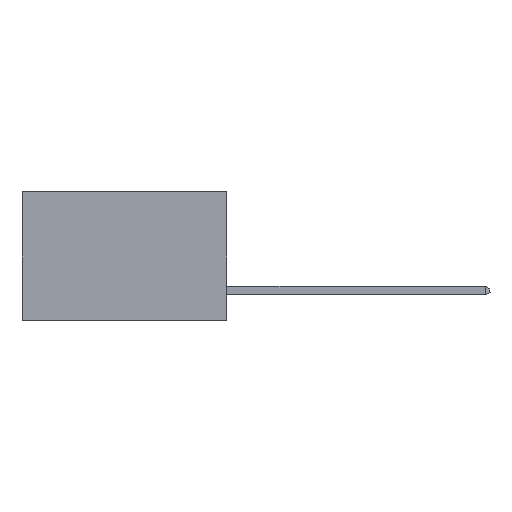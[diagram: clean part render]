
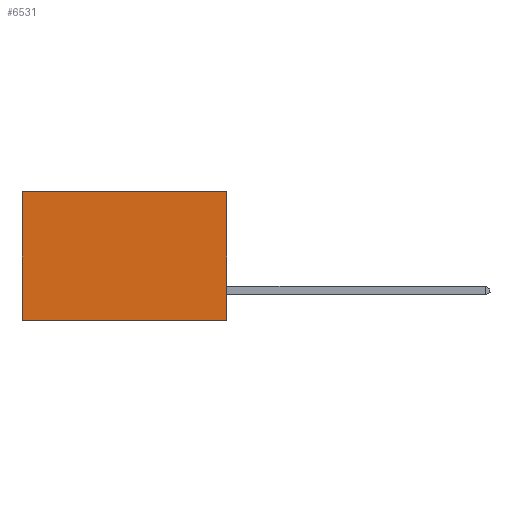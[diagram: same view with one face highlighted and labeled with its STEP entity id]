
A CAD part, left-side view. The second image highlights one B-rep face of the part: STEP entity #6531.
In plain terms, the highlighted planar face has unit normal (-1, 0, 0).
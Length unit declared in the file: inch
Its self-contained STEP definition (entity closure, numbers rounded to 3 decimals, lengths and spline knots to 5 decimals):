
#491 = EDGE_CURVE ( 'NONE', #18198, #8046, #5920, .T. ) ;
#566 = ORIENTED_EDGE ( 'NONE', *, *, #17327, .T. ) ;
#859 = ORIENTED_EDGE ( 'NONE', *, *, #15219, .F. ) ;
#930 = ORIENTED_EDGE ( 'NONE', *, *, #10000, .F. ) ;
#2022 = ORIENTED_EDGE ( 'NONE', *, *, #491, .T. ) ;
#2604 = EDGE_LOOP ( 'NONE', ( #566, #859, #930, #2022 ) ) ;
#4868 = PLANE ( 'NONE',  #19497 ) ;
#5141 = DIRECTION ( 'NONE',  ( 1., 0., 0. ) ) ;
#5213 = CARTESIAN_POINT ( 'NONE',  ( 0.277, 0., 0. ) ) ;
#5254 = CARTESIAN_POINT ( 'NONE',  ( 0.277, 0., -0.37 ) ) ;
#5471 = DIRECTION ( 'NONE',  ( 0., 0., -1. ) ) ;
#5523 = CARTESIAN_POINT ( 'NONE',  ( 0.277, 0., -0.37 ) ) ;
#5920 = LINE ( 'NONE', #11319, #9643 ) ;
#5972 = VERTEX_POINT ( 'NONE', #17853 ) ;
#6531 = ADVANCED_FACE ( 'NONE', ( #9197 ), #4868, .F. ) ;
#8046 = VERTEX_POINT ( 'NONE', #18456 ) ;
#8834 = LINE ( 'NONE', #5523, #16611 ) ;
#9197 = FACE_OUTER_BOUND ( 'NONE', #2604, .T. ) ;
#9580 = VERTEX_POINT ( 'NONE', #18432 ) ;
#9643 = VECTOR ( 'NONE', #19294, 39.37008 ) ;
#10000 = EDGE_CURVE ( 'NONE', #18198, #5972, #8834, .T. ) ;
#11319 = CARTESIAN_POINT ( 'NONE',  ( 0.277, 0., 0. ) ) ;
#12014 = LINE ( 'NONE', #19962, #19624 ) ;
#13278 = VECTOR ( 'NONE', #16292, 39.37008 ) ;
#13936 = DIRECTION ( 'NONE',  ( 0., 0., -1. ) ) ;
#15219 = EDGE_CURVE ( 'NONE', #5972, #9580, #17357, .T. ) ;
#16292 = DIRECTION ( 'NONE',  ( 0., 1., 0. ) ) ;
#16352 = CARTESIAN_POINT ( 'NONE',  ( 0.277, 0., -0.37 ) ) ;
#16476 = DIRECTION ( 'NONE',  ( 0., 0., -1. ) ) ;
#16611 = VECTOR ( 'NONE', #16476, 39.37008 ) ;
#17327 = EDGE_CURVE ( 'NONE', #8046, #9580, #12014, .T. ) ;
#17357 = LINE ( 'NONE', #16352, #13278 ) ;
#17853 = CARTESIAN_POINT ( 'NONE',  ( 0.277, 0., -0.37 ) ) ;
#18198 = VERTEX_POINT ( 'NONE', #5213 ) ;
#18432 = CARTESIAN_POINT ( 'NONE',  ( 0.277, 0.59, -0.37 ) ) ;
#18456 = CARTESIAN_POINT ( 'NONE',  ( 0.277, 0.59, 0. ) ) ;
#19294 = DIRECTION ( 'NONE',  ( 0., 1., 0. ) ) ;
#19497 = AXIS2_PLACEMENT_3D ( 'NONE', #5254, #5141, #5471 ) ;
#19624 = VECTOR ( 'NONE', #13936, 39.37008 ) ;
#19962 = CARTESIAN_POINT ( 'NONE',  ( 0.277, 0.59, -0.37 ) ) ;
